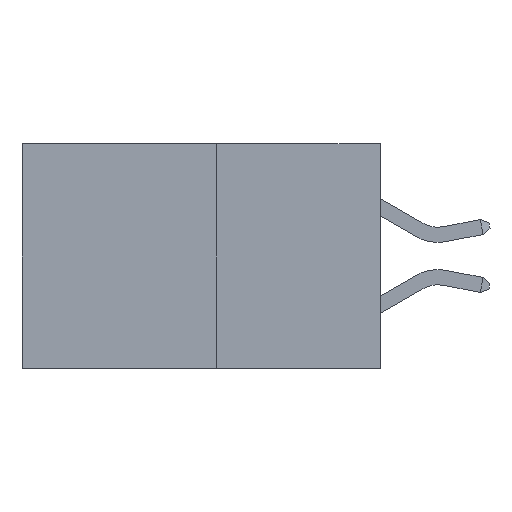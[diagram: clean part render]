
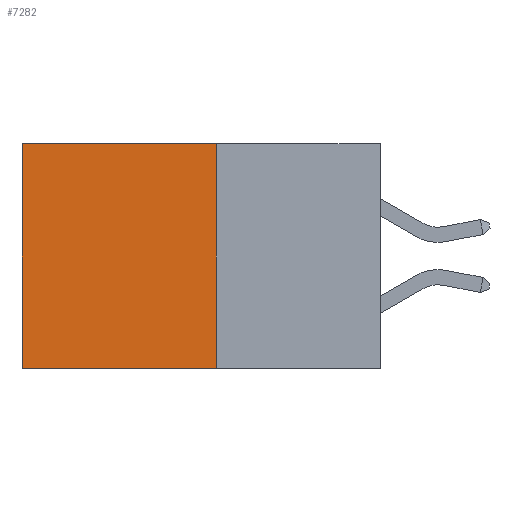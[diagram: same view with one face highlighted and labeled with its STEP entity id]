
A CAD part, left-side view. The second image highlights one B-rep face of the part: STEP entity #7282.
In plain terms, the highlighted planar face has unit normal (-1, 0, 0).
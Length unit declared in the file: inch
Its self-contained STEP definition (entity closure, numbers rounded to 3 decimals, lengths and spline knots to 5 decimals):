
#203 = LINE ( 'NONE', #1902, #11785 ) ;
#473 = CARTESIAN_POINT ( 'NONE',  ( 0.277, 0.59, 0. ) ) ;
#592 = DIRECTION ( 'NONE',  ( 0., 0., -1. ) ) ;
#1514 = EDGE_CURVE ( 'NONE', #10617, #11040, #1928, .T. ) ;
#1592 = LINE ( 'NONE', #6417, #8755 ) ;
#1902 = CARTESIAN_POINT ( 'NONE',  ( 0.277, 0.59, -0.37 ) ) ;
#1928 = LINE ( 'NONE', #3030, #2239 ) ;
#2116 = AXIS2_PLACEMENT_3D ( 'NONE', #10860, #8351, #2824 ) ;
#2239 = VECTOR ( 'NONE', #2872, 39.37008 ) ;
#2483 = ORIENTED_EDGE ( 'NONE', *, *, #6512, .T. ) ;
#2778 = EDGE_LOOP ( 'NONE', ( #5409, #11788, #5683, #2483 ) ) ;
#2824 = DIRECTION ( 'NONE',  ( 0., 0., -1. ) ) ;
#2872 = DIRECTION ( 'NONE',  ( 0., 1., 0. ) ) ;
#3030 = CARTESIAN_POINT ( 'NONE',  ( 0.277, 0.27, -0.37 ) ) ;
#3654 = EDGE_CURVE ( 'NONE', #11792, #10617, #1592, .T. ) ;
#5031 = CARTESIAN_POINT ( 'NONE',  ( 0.277, 0.27, 0. ) ) ;
#5409 = ORIENTED_EDGE ( 'NONE', *, *, #6696, .T. ) ;
#5683 = ORIENTED_EDGE ( 'NONE', *, *, #3654, .F. ) ;
#5691 = DIRECTION ( 'NONE',  ( 0., 1., 0. ) ) ;
#5824 = DIRECTION ( 'NONE',  ( 0., 0., -1. ) ) ;
#6054 = FACE_OUTER_BOUND ( 'NONE', #2778, .T. ) ;
#6334 = LINE ( 'NONE', #10003, #8403 ) ;
#6417 = CARTESIAN_POINT ( 'NONE',  ( 0.277, 0.27, -0.37 ) ) ;
#6512 = EDGE_CURVE ( 'NONE', #11792, #11153, #6334, .T. ) ;
#6562 = PLANE ( 'NONE',  #2116 ) ;
#6696 = EDGE_CURVE ( 'NONE', #11153, #11040, #203, .T. ) ;
#7282 = ADVANCED_FACE ( 'NONE', ( #6054 ), #6562, .F. ) ;
#8351 = DIRECTION ( 'NONE',  ( 1., 0., 0. ) ) ;
#8403 = VECTOR ( 'NONE', #5691, 39.37008 ) ;
#8755 = VECTOR ( 'NONE', #592, 39.37008 ) ;
#9423 = CARTESIAN_POINT ( 'NONE',  ( 0.277, 0.27, -0.37 ) ) ;
#9719 = CARTESIAN_POINT ( 'NONE',  ( 0.277, 0.59, -0.37 ) ) ;
#10003 = CARTESIAN_POINT ( 'NONE',  ( 0.277, 0.27, 0. ) ) ;
#10617 = VERTEX_POINT ( 'NONE', #9423 ) ;
#10860 = CARTESIAN_POINT ( 'NONE',  ( 0.277, 0.27, -0.37 ) ) ;
#11040 = VERTEX_POINT ( 'NONE', #9719 ) ;
#11153 = VERTEX_POINT ( 'NONE', #473 ) ;
#11785 = VECTOR ( 'NONE', #5824, 39.37008 ) ;
#11788 = ORIENTED_EDGE ( 'NONE', *, *, #1514, .F. ) ;
#11792 = VERTEX_POINT ( 'NONE', #5031 ) ;
